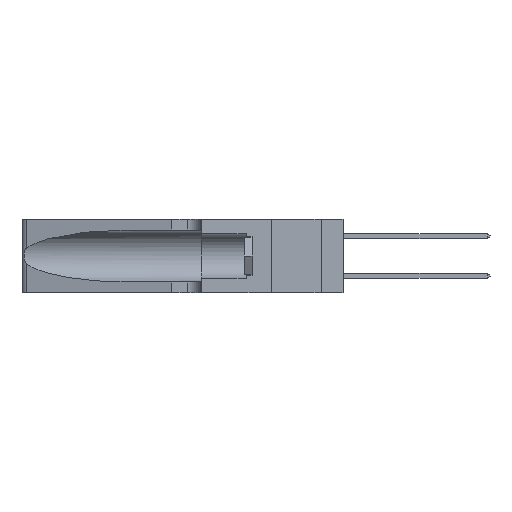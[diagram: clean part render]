
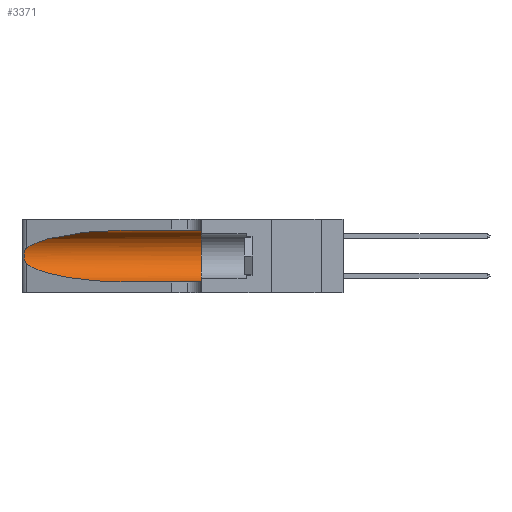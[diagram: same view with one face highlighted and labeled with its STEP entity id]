
A CAD part, left-side view. The second image highlights one B-rep face of the part: STEP entity #3371.
In plain terms, the highlighted cylindrical face has radius 3.308 mm (diameter 6.617 mm), a partial arc.
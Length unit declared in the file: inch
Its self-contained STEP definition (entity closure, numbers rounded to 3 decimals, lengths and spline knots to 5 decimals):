
#77 = EDGE_CURVE ( 'NONE', #19304, #33784, #30745, .T. ) ;
#1253 =( BOUNDED_CURVE ( )  B_SPLINE_CURVE ( 3, ( #19633, #36846, #25452, #8212 ),
 .UNSPECIFIED., .F., .F. ) 
 B_SPLINE_CURVE_WITH_KNOTS ( ( 4, 4 ),
 ( 3.44316, 4.71239 ),
 .UNSPECIFIED. ) 
 CURVE ( )  GEOMETRIC_REPRESENTATION_ITEM ( )  RATIONAL_B_SPLINE_CURVE ( ( 1., 0.87, 0.87, 1. ) ) 
 REPRESENTATION_ITEM ( '' )  );
#1352 = CARTESIAN_POINT ( 'NONE',  ( 0.25555, 1.22994, 0.2215 ) ) ;
#1479 = CARTESIAN_POINT ( 'NONE',  ( 0.26075, 1.23896, 0.178 ) ) ;
#2118 = EDGE_CURVE ( 'NONE', #35371, #19017, #16243, .T. ) ;
#3371 = ADVANCED_FACE ( 'NONE', ( #35042 ), #11217, .F. ) ;
#3398 = DIRECTION ( 'NONE',  ( 0., -1., 0. ) ) ;
#3430 = EDGE_CURVE ( 'NONE', #33784, #23819, #24081, .T. ) ;
#3856 = CARTESIAN_POINT ( 'NONE',  ( 0.1305, 1.61858, 0.185 ) ) ;
#4350 = CARTESIAN_POINT ( 'NONE',  ( 0.25856, 1.23593, 0.16098 ) ) ;
#4422 = ORIENTED_EDGE ( 'NONE', *, *, #77, .T. ) ;
#4901 = ORIENTED_EDGE ( 'NONE', *, *, #2118, .F. ) ;
#6205 = LINE ( 'NONE', #35441, #21506 ) ;
#7235 = DIRECTION ( 'NONE',  ( 0., 1., 0. ) ) ;
#7274 = CARTESIAN_POINT ( 'NONE',  ( 0.25639, 1.23186, 0.15144 ) ) ;
#8212 = CARTESIAN_POINT ( 'NONE',  ( 0.1305, 0.72297, 0.05475 ) ) ;
#10160 = CARTESIAN_POINT ( 'NONE',  ( 0.25487, 1.22718, 0.14631 ) ) ;
#11217 = CYLINDRICAL_SURFACE ( 'NONE', #13389, 0.13025 ) ;
#12009 = CARTESIAN_POINT ( 'NONE',  ( 0.1305, 0.35, 0.31525 ) ) ;
#12540 = DIRECTION ( 'NONE',  ( 0., -1., 0. ) ) ;
#12807 = VERTEX_POINT ( 'NONE', #23734 ) ;
#12907 = CARTESIAN_POINT ( 'NONE',  ( 0.25639, 1.23184, 0.21858 ) ) ;
#13389 = AXIS2_PLACEMENT_3D ( 'NONE', #3856, #12540, #21099 ) ;
#14005 = EDGE_CURVE ( 'NONE', #19304, #35371, #32558, .T. ) ;
#15348 = DIRECTION ( 'NONE',  ( 0., -1., 0. ) ) ;
#15794 = CARTESIAN_POINT ( 'NONE',  ( 0.25854, 1.2359, 0.20912 ) ) ;
#16243 = CIRCLE ( 'NONE', #31664, 0.13025 ) ;
#18409 = ORIENTED_EDGE ( 'NONE', *, *, #20282, .T. ) ;
#18708 = CARTESIAN_POINT ( 'NONE',  ( 0.26075, 1.23896, 0.19203 ) ) ;
#19017 = VERTEX_POINT ( 'NONE', #36026 ) ;
#19304 = VERTEX_POINT ( 'NONE', #28735 ) ;
#19633 = CARTESIAN_POINT ( 'NONE',  ( 0.25487, 1.22718, 0.14631 ) ) ;
#20282 = EDGE_CURVE ( 'NONE', #12807, #19017, #6205, .T. ) ;
#20630 = CARTESIAN_POINT ( 'NONE',  ( 0.1305, 1.61858, 0.31525 ) ) ;
#21099 = DIRECTION ( 'NONE',  ( 0., 0., -1. ) ) ;
#21506 = VECTOR ( 'NONE', #15348, 39.37008 ) ;
#21539 = ORIENTED_EDGE ( 'NONE', *, *, #28019, .T. ) ;
#21597 = CARTESIAN_POINT ( 'NONE',  ( 0.26017, 1.23833, 0.17102 ) ) ;
#23576 = CARTESIAN_POINT ( 'NONE',  ( 0.1305, 0.72297, 0.31525 ) ) ;
#23734 = CARTESIAN_POINT ( 'NONE',  ( 0.1305, 0.72297, 0.05475 ) ) ;
#23819 = VERTEX_POINT ( 'NONE', #30395 ) ;
#24081 = B_SPLINE_CURVE_WITH_KNOTS ( 'NONE', 3,
 ( #27275, #1352, #12907, #33029, #15794, #35895, #18708, #1479, #21597, #4350, #24511, #7274, #27393, #10160 ),
 .UNSPECIFIED., .F., .F.,
 ( 4, 2, 2, 2, 2, 2, 4 ),
 ( 0., 0.00027, 0.00053, 0.00107, 0.0016, 0.00187, 0.00214 ),
 .UNSPECIFIED. ) ;
#24476 = CARTESIAN_POINT ( 'NONE',  ( 0.1305, 0.35, 0.185 ) ) ;
#24511 = CARTESIAN_POINT ( 'NONE',  ( 0.25789, 1.23486, 0.15765 ) ) ;
#25452 = CARTESIAN_POINT ( 'NONE',  ( 0.18966, 0.96281, 0.05475 ) ) ;
#25780 = CARTESIAN_POINT ( 'NONE',  ( 0.2373, 1.15595, 0.28018 ) ) ;
#27275 = CARTESIAN_POINT ( 'NONE',  ( 0.25487, 1.22718, 0.22369 ) ) ;
#27359 = DIRECTION ( 'NONE',  ( 0., 0., 1. ) ) ;
#27393 = CARTESIAN_POINT ( 'NONE',  ( 0.25555, 1.22993, 0.14849 ) ) ;
#27403 = ORIENTED_EDGE ( 'NONE', *, *, #3430, .T. ) ;
#27865 = ORIENTED_EDGE ( 'NONE', *, *, #14005, .F. ) ;
#28019 = EDGE_CURVE ( 'NONE', #23819, #12807, #1253, .T. ) ;
#28735 = CARTESIAN_POINT ( 'NONE',  ( 0.1305, 0.72297, 0.31525 ) ) ;
#29388 = CARTESIAN_POINT ( 'NONE',  ( 0.18966, 0.96281, 0.31525 ) ) ;
#30395 = CARTESIAN_POINT ( 'NONE',  ( 0.25487, 1.22718, 0.14631 ) ) ;
#30745 =( BOUNDED_CURVE ( )  B_SPLINE_CURVE ( 3, ( #23576, #29388, #25780, #36823 ),
 .UNSPECIFIED., .F., .F. ) 
 B_SPLINE_CURVE_WITH_KNOTS ( ( 4, 4 ),
 ( 1.5708, 2.84003 ),
 .UNSPECIFIED. ) 
 CURVE ( )  GEOMETRIC_REPRESENTATION_ITEM ( )  RATIONAL_B_SPLINE_CURVE ( ( 1., 0.87, 0.87, 1. ) ) 
 REPRESENTATION_ITEM ( '' )  );
#31654 = VECTOR ( 'NONE', #3398, 39.37008 ) ;
#31664 = AXIS2_PLACEMENT_3D ( 'NONE', #24476, #7235, #27359 ) ;
#32099 = EDGE_LOOP ( 'NONE', ( #4422, #27403, #21539, #18409, #4901, #27865 ) ) ;
#32429 = CARTESIAN_POINT ( 'NONE',  ( 0.25487, 1.22718, 0.22369 ) ) ;
#32558 = LINE ( 'NONE', #20630, #31654 ) ;
#33029 = CARTESIAN_POINT ( 'NONE',  ( 0.25787, 1.23484, 0.2124 ) ) ;
#33784 = VERTEX_POINT ( 'NONE', #32429 ) ;
#35042 = FACE_OUTER_BOUND ( 'NONE', #32099, .T. ) ;
#35371 = VERTEX_POINT ( 'NONE', #12009 ) ;
#35441 = CARTESIAN_POINT ( 'NONE',  ( 0.1305, 1.61858, 0.05475 ) ) ;
#35895 = CARTESIAN_POINT ( 'NONE',  ( 0.26018, 1.23835, 0.19895 ) ) ;
#36026 = CARTESIAN_POINT ( 'NONE',  ( 0.1305, 0.35, 0.05475 ) ) ;
#36823 = CARTESIAN_POINT ( 'NONE',  ( 0.25487, 1.22718, 0.22369 ) ) ;
#36846 = CARTESIAN_POINT ( 'NONE',  ( 0.2373, 1.15595, 0.08982 ) ) ;
